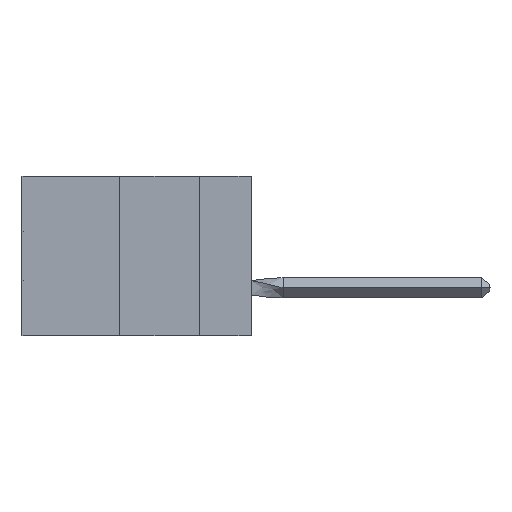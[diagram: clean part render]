
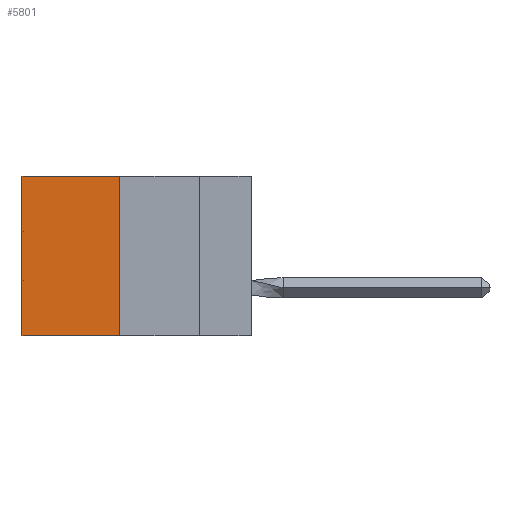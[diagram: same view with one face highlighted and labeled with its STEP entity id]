
A CAD part, left-side view. The second image highlights one B-rep face of the part: STEP entity #5801.
In plain terms, the highlighted planar face has unit normal (-1, 0, 0).
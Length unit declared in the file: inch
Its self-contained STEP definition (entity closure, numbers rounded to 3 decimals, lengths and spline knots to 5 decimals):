
#5801 = ADVANCED_FACE ( 'NONE', ( #39357 ), #29456, .F. ) ;
#7329 = EDGE_CURVE ( 'NONE', #12737, #30275, #25291, .T. ) ;
#8358 = EDGE_LOOP ( 'NONE', ( #9462, #27602, #31305, #14761 ) ) ;
#9462 = ORIENTED_EDGE ( 'NONE', *, *, #40528, .T. ) ;
#10044 = VECTOR ( 'NONE', #41082, 39.37008 ) ;
#10941 = EDGE_CURVE ( 'NONE', #30275, #39135, #26449, .T. ) ;
#11663 = DIRECTION ( 'NONE',  ( 0., 0., -1. ) ) ;
#12737 = VERTEX_POINT ( 'NONE', #15761 ) ;
#12956 = VERTEX_POINT ( 'NONE', #41128 ) ;
#14761 = ORIENTED_EDGE ( 'NONE', *, *, #24769, .T. ) ;
#14869 = CARTESIAN_POINT ( 'NONE',  ( 0.305, 0.413, -0.5 ) ) ;
#15761 = CARTESIAN_POINT ( 'NONE',  ( 0.305, 0.413, 0. ) ) ;
#15925 = VECTOR ( 'NONE', #11663, 39.37008 ) ;
#21289 = CARTESIAN_POINT ( 'NONE',  ( 0.305, 0.72, -0.5 ) ) ;
#21811 = VECTOR ( 'NONE', #23495, 39.37008 ) ;
#23013 = CARTESIAN_POINT ( 'NONE',  ( 0.305, 0.72, -0.5 ) ) ;
#23495 = DIRECTION ( 'NONE',  ( 0., 1., 0. ) ) ;
#24769 = EDGE_CURVE ( 'NONE', #12737, #12956, #31652, .T. ) ;
#25291 = LINE ( 'NONE', #14869, #15925 ) ;
#26449 = LINE ( 'NONE', #27860, #39853 ) ;
#26532 = AXIS2_PLACEMENT_3D ( 'NONE', #32964, #26857, #33399 ) ;
#26824 = CARTESIAN_POINT ( 'NONE',  ( 0.305, 0.413, 0. ) ) ;
#26857 = DIRECTION ( 'NONE',  ( 1., 0., 0. ) ) ;
#27602 = ORIENTED_EDGE ( 'NONE', *, *, #10941, .F. ) ;
#27860 = CARTESIAN_POINT ( 'NONE',  ( 0.305, 0.413, -0.5 ) ) ;
#29456 = PLANE ( 'NONE',  #26532 ) ;
#30275 = VERTEX_POINT ( 'NONE', #40994 ) ;
#31305 = ORIENTED_EDGE ( 'NONE', *, *, #7329, .F. ) ;
#31652 = LINE ( 'NONE', #26824, #21811 ) ;
#32964 = CARTESIAN_POINT ( 'NONE',  ( 0.305, 0.413, -0.5 ) ) ;
#33399 = DIRECTION ( 'NONE',  ( 0., 0., -1. ) ) ;
#34843 = DIRECTION ( 'NONE',  ( 0., 1., 0. ) ) ;
#39135 = VERTEX_POINT ( 'NONE', #23013 ) ;
#39357 = FACE_OUTER_BOUND ( 'NONE', #8358, .T. ) ;
#39853 = VECTOR ( 'NONE', #34843, 39.37008 ) ;
#40528 = EDGE_CURVE ( 'NONE', #12956, #39135, #41147, .T. ) ;
#40994 = CARTESIAN_POINT ( 'NONE',  ( 0.305, 0.413, -0.5 ) ) ;
#41082 = DIRECTION ( 'NONE',  ( 0., 0., -1. ) ) ;
#41128 = CARTESIAN_POINT ( 'NONE',  ( 0.305, 0.72, 0. ) ) ;
#41147 = LINE ( 'NONE', #21289, #10044 ) ;
